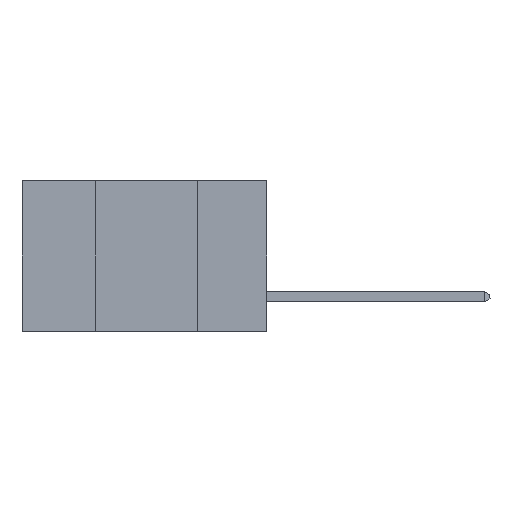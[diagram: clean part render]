
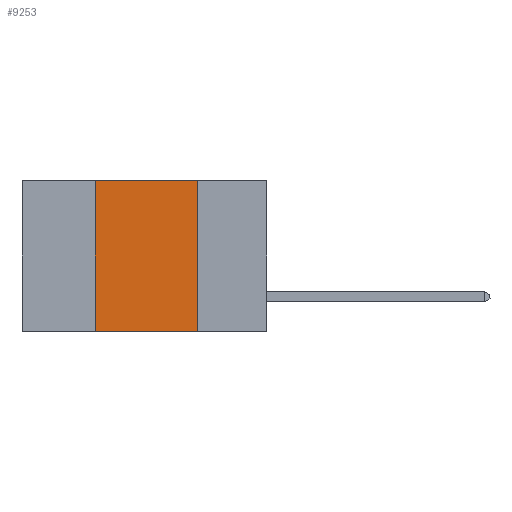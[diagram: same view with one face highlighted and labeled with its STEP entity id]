
A CAD part, left-side view. The second image highlights one B-rep face of the part: STEP entity #9253.
In plain terms, the highlighted planar face has unit normal (-1, 0, 0).
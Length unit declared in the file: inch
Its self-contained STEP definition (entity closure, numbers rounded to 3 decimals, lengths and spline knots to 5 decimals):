
#258 = PLANE ( 'NONE',  #5746 ) ;
#453 = EDGE_CURVE ( 'NONE', #4787, #5967, #12351, .T. ) ;
#461 = ORIENTED_EDGE ( 'NONE', *, *, #10067, .F. ) ;
#1817 = VERTEX_POINT ( 'NONE', #9082 ) ;
#2423 = CARTESIAN_POINT ( 'NONE',  ( 0., 0.17, -0.37 ) ) ;
#2478 = CARTESIAN_POINT ( 'NONE',  ( 0., 0.42, 0. ) ) ;
#2577 = CARTESIAN_POINT ( 'NONE',  ( 0., 0.6, -0.37 ) ) ;
#2618 = DIRECTION ( 'NONE',  ( 0., -1., 0. ) ) ;
#3032 = ORIENTED_EDGE ( 'NONE', *, *, #5567, .F. ) ;
#3185 = LINE ( 'NONE', #2577, #10668 ) ;
#3339 = ORIENTED_EDGE ( 'NONE', *, *, #5990, .T. ) ;
#3366 = DIRECTION ( 'NONE',  ( 0., 0., -1. ) ) ;
#3740 = DIRECTION ( 'NONE',  ( 0., -1., 0. ) ) ;
#3867 = CARTESIAN_POINT ( 'NONE',  ( 0., 0.42, 0. ) ) ;
#4505 = EDGE_LOOP ( 'NONE', ( #13077, #3032, #461, #3339 ) ) ;
#4685 = CARTESIAN_POINT ( 'NONE',  ( 0., 0.17, 0. ) ) ;
#4787 = VERTEX_POINT ( 'NONE', #6492 ) ;
#5235 = VECTOR ( 'NONE', #3366, 39.37008 ) ;
#5243 = LINE ( 'NONE', #5606, #12932 ) ;
#5529 = DIRECTION ( 'NONE',  ( 1., 0., 0. ) ) ;
#5567 = EDGE_CURVE ( 'NONE', #8929, #4787, #5243, .T. ) ;
#5606 = CARTESIAN_POINT ( 'NONE',  ( 0., 0.6, 0. ) ) ;
#5746 = AXIS2_PLACEMENT_3D ( 'NONE', #11618, #5529, #12556 ) ;
#5967 = VERTEX_POINT ( 'NONE', #2423 ) ;
#5990 = EDGE_CURVE ( 'NONE', #1817, #5967, #3185, .T. ) ;
#6492 = CARTESIAN_POINT ( 'NONE',  ( 0., 0.17, 0. ) ) ;
#7348 = FACE_OUTER_BOUND ( 'NONE', #4505, .T. ) ;
#7586 = VECTOR ( 'NONE', #12573, 39.37008 ) ;
#8929 = VERTEX_POINT ( 'NONE', #3867 ) ;
#9082 = CARTESIAN_POINT ( 'NONE',  ( 0., 0.42, -0.37 ) ) ;
#9253 = ADVANCED_FACE ( 'NONE', ( #7348 ), #258, .F. ) ;
#10067 = EDGE_CURVE ( 'NONE', #1817, #8929, #10629, .T. ) ;
#10629 = LINE ( 'NONE', #2478, #7586 ) ;
#10668 = VECTOR ( 'NONE', #2618, 39.37008 ) ;
#11618 = CARTESIAN_POINT ( 'NONE',  ( 0., 0.6, 0. ) ) ;
#12351 = LINE ( 'NONE', #4685, #5235 ) ;
#12556 = DIRECTION ( 'NONE',  ( 0., 0., -1. ) ) ;
#12573 = DIRECTION ( 'NONE',  ( 0., 0., 1. ) ) ;
#12932 = VECTOR ( 'NONE', #3740, 39.37008 ) ;
#13077 = ORIENTED_EDGE ( 'NONE', *, *, #453, .F. ) ;
